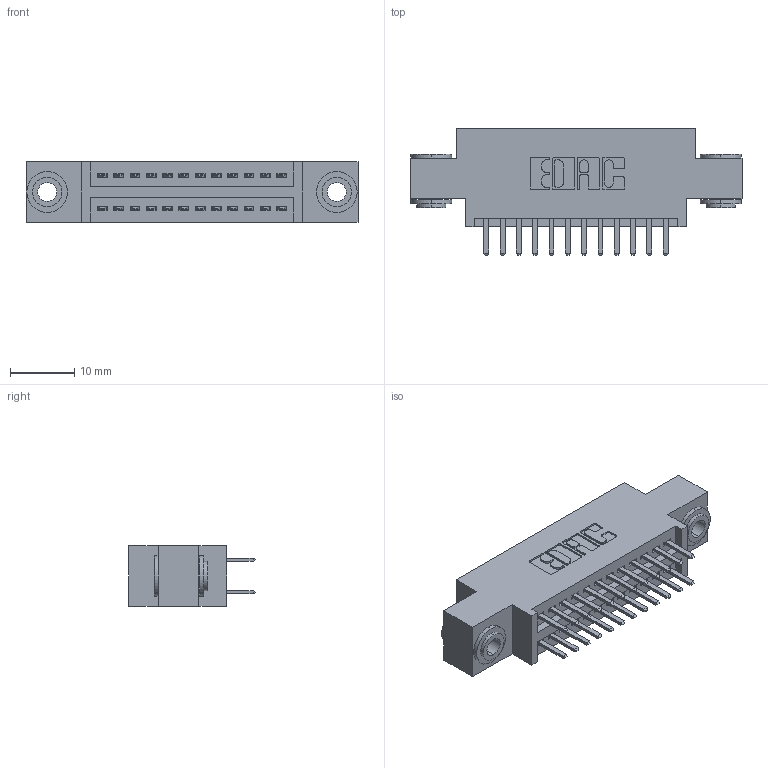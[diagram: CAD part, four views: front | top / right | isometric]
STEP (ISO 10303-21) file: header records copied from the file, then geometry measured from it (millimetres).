
FILE_DESCRIPTION (( 'STEP AP203' ), '1' );
FILE_NAME ('395-024-520-803.STEP', '2019-10-16T15:53:03', ( '' ), ( '' ), 'SwSTEP 2.0', 'SolidWorks 2016', '' );
FILE_SCHEMA (( 'CONFIG_CONTROL_DESIGN' ));
Length unit declared in the file: inch
Products named in the file (4): 345 Part_0.170 Offset - 0.156 Dia-TH; 345-292-001_345-293-120; 345-250-002_345-250-002-102; 395-024-520-803
Assembly tree (27 placements, depth 2):
  395-024-520-803
    345 Part_0.170 Offset - 0.156 Dia-TH
    345-292-001_345-293-120  x24
    345-250-002_345-250-002-102  x2
Bounding box: 51.69 x 19.68 x 9.4 mm (x, y, z)
Volume: 4638.1 mm3; surface area: 6600.8 mm2
Topology: 27 solids, 27 shells, 1464 faces, 4197 edges, 2730 vertices
Faces by surface type: plane 934, cylinder 522, cone 8
Entity records: 14350 total; most frequent: CARTESIAN_POINT 2423, ORIENTED_EDGE 2338, DIRECTION 2191, EDGE_CURVE 1169, VECTOR 961, LINE 961, VERTEX_POINT 774, AXIS2_PLACEMENT_3D 615
